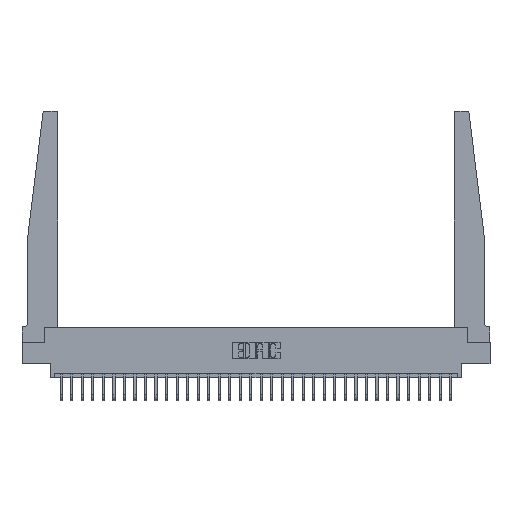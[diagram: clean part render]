
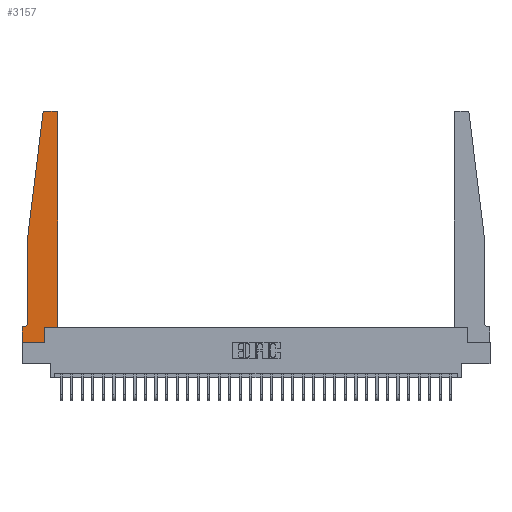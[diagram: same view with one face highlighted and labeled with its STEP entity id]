
A CAD part, top view. The second image highlights one B-rep face of the part: STEP entity #3157.
In plain terms, the highlighted planar face has unit normal (0, 0, 1).
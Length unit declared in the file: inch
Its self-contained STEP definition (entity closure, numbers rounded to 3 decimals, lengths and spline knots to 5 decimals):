
#404 = EDGE_CURVE ( 'NONE', #16977, #12662, #30665, .T. ) ;
#1570 = CIRCLE ( 'NONE', #20117, 0.05 ) ;
#1649 = CARTESIAN_POINT ( 'NONE',  ( 0.065, 0.2375, 0.37 ) ) ;
#1720 = CARTESIAN_POINT ( 'NONE',  ( 0.015, 0.2375, 0.37 ) ) ;
#2213 = CARTESIAN_POINT ( 'NONE',  ( 0., 0., 0.37 ) ) ;
#2411 = VECTOR ( 'NONE', #4899, 39.37008 ) ;
#2542 = ORIENTED_EDGE ( 'NONE', *, *, #15255, .T. ) ;
#2802 = EDGE_CURVE ( 'NONE', #7478, #3315, #29789, .T. ) ;
#3157 = ADVANCED_FACE ( 'NONE', ( #14568 ), #27684, .T. ) ;
#3315 = VERTEX_POINT ( 'NONE', #20793 ) ;
#3587 = DIRECTION ( 'NONE',  ( 0., 0., 1. ) ) ;
#3702 = VERTEX_POINT ( 'NONE', #26101 ) ;
#4328 = CARTESIAN_POINT ( 'NONE',  ( 0., 0.1875, 0.37 ) ) ;
#4753 = CARTESIAN_POINT ( 'NONE',  ( 0.065, 1.25, 0.37 ) ) ;
#4840 = VERTEX_POINT ( 'NONE', #12792 ) ;
#4899 = DIRECTION ( 'NONE',  ( -1., 0., 0. ) ) ;
#5077 = CARTESIAN_POINT ( 'NONE',  ( 0., 0.1875, 0.37 ) ) ;
#5295 = AXIS2_PLACEMENT_3D ( 'NONE', #22909, #23234, #8042 ) ;
#5657 = VERTEX_POINT ( 'NONE', #15448 ) ;
#6003 = LINE ( 'NONE', #20778, #17281 ) ;
#6250 = ORIENTED_EDGE ( 'NONE', *, *, #30817, .T. ) ;
#6309 = CARTESIAN_POINT ( 'NONE',  ( 0.27653, 2.72, 0.37 ) ) ;
#7261 = DIRECTION ( 'NONE',  ( 0., -1., 0. ) ) ;
#7462 = DIRECTION ( 'NONE',  ( 1., 0., 0. ) ) ;
#7478 = VERTEX_POINT ( 'NONE', #13219 ) ;
#8042 = DIRECTION ( 'NONE',  ( 1., 0., 0. ) ) ;
#9351 = EDGE_CURVE ( 'NONE', #14715, #16769, #27102, .T. ) ;
#9834 = VECTOR ( 'NONE', #16742, 39.37008 ) ;
#9995 = EDGE_CURVE ( 'NONE', #16769, #20593, #6003, .T. ) ;
#10140 = EDGE_CURVE ( 'NONE', #5657, #4840, #31924, .T. ) ;
#10900 = DIRECTION ( 'NONE',  ( 1., 0., 0. ) ) ;
#11083 = CARTESIAN_POINT ( 'NONE',  ( 0.425, 0.18, 0.37 ) ) ;
#11259 = ORIENTED_EDGE ( 'NONE', *, *, #29281, .T. ) ;
#11339 = ORIENTED_EDGE ( 'NONE', *, *, #404, .T. ) ;
#12044 = CIRCLE ( 'NONE', #19406, 0.03 ) ;
#12596 = VECTOR ( 'NONE', #30303, 39.37008 ) ;
#12662 = VERTEX_POINT ( 'NONE', #26445 ) ;
#12791 = DIRECTION ( 'NONE',  ( 0., 0., 1. ) ) ;
#12792 = CARTESIAN_POINT ( 'NONE',  ( 0.27653, 2.75, 0.37 ) ) ;
#12931 = CARTESIAN_POINT ( 'NONE',  ( 0.2605, 0.18, 0.37 ) ) ;
#12933 = DIRECTION ( 'NONE',  ( 0., -1., 0. ) ) ;
#13214 = EDGE_LOOP ( 'NONE', ( #26716, #2542, #11339, #28856, #30736, #14080, #29726, #18255, #19388, #6250, #16619, #11259 ) ) ;
#13219 = CARTESIAN_POINT ( 'NONE',  ( 0.425, 0.18, 0.37 ) ) ;
#13433 = VECTOR ( 'NONE', #19831, 39.37008 ) ;
#14080 = ORIENTED_EDGE ( 'NONE', *, *, #23127, .T. ) ;
#14568 = FACE_OUTER_BOUND ( 'NONE', #13214, .T. ) ;
#14636 = LINE ( 'NONE', #30090, #21653 ) ;
#14645 = CARTESIAN_POINT ( 'NONE',  ( 0.065, 0.1875, 0.37 ) ) ;
#14715 = VERTEX_POINT ( 'NONE', #4328 ) ;
#15255 = EDGE_CURVE ( 'NONE', #4840, #16977, #12044, .T. ) ;
#15448 = CARTESIAN_POINT ( 'NONE',  ( 0.395, 2.75, 0.37 ) ) ;
#15822 = AXIS2_PLACEMENT_3D ( 'NONE', #5077, #12791, #7462 ) ;
#15834 = DIRECTION ( 'NONE',  ( 1., 0., 0. ) ) ;
#15869 = VECTOR ( 'NONE', #15834, 39.37008 ) ;
#16035 = LINE ( 'NONE', #12931, #12596 ) ;
#16619 = ORIENTED_EDGE ( 'NONE', *, *, #2802, .T. ) ;
#16742 = DIRECTION ( 'NONE',  ( -1., 0., 0. ) ) ;
#16769 = VERTEX_POINT ( 'NONE', #18659 ) ;
#16977 = VERTEX_POINT ( 'NONE', #29431 ) ;
#17281 = VECTOR ( 'NONE', #23282, 39.37008 ) ;
#17885 = CIRCLE ( 'NONE', #5295, 0.03 ) ;
#18255 = ORIENTED_EDGE ( 'NONE', *, *, #9995, .T. ) ;
#18659 = CARTESIAN_POINT ( 'NONE',  ( 0., 0., 0.37 ) ) ;
#19321 = EDGE_CURVE ( 'NONE', #12662, #21809, #14636, .T. ) ;
#19388 = ORIENTED_EDGE ( 'NONE', *, *, #21782, .T. ) ;
#19406 = AXIS2_PLACEMENT_3D ( 'NONE', #6309, #3587, #10900 ) ;
#19831 = DIRECTION ( 'NONE',  ( 0., 1., 0. ) ) ;
#20117 = AXIS2_PLACEMENT_3D ( 'NONE', #1720, #31508, #28956 ) ;
#20463 = CARTESIAN_POINT ( 'NONE',  ( 0.2605, 0.18, 0.37 ) ) ;
#20593 = VERTEX_POINT ( 'NONE', #25349 ) ;
#20778 = CARTESIAN_POINT ( 'NONE',  ( 0., 0., 0.37 ) ) ;
#20793 = CARTESIAN_POINT ( 'NONE',  ( 0.425, 2.72, 0.37 ) ) ;
#21653 = VECTOR ( 'NONE', #12933, 39.37008 ) ;
#21782 = EDGE_CURVE ( 'NONE', #20593, #32049, #16035, .T. ) ;
#21809 = VERTEX_POINT ( 'NONE', #1649 ) ;
#22492 = LINE ( 'NONE', #11083, #15869 ) ;
#22909 = CARTESIAN_POINT ( 'NONE',  ( 0.395, 2.72, 0.37 ) ) ;
#23127 = EDGE_CURVE ( 'NONE', #3702, #14715, #23728, .T. ) ;
#23234 = DIRECTION ( 'NONE',  ( 0., 0., 1. ) ) ;
#23282 = DIRECTION ( 'NONE',  ( 1., 0., 0. ) ) ;
#23728 = LINE ( 'NONE', #14645, #2411 ) ;
#24320 = VECTOR ( 'NONE', #7261, 39.37008 ) ;
#24478 = VECTOR ( 'NONE', #28370, 39.37008 ) ;
#25349 = CARTESIAN_POINT ( 'NONE',  ( 0.2605, 0., 0.37 ) ) ;
#26101 = CARTESIAN_POINT ( 'NONE',  ( 0.015, 0.1875, 0.37 ) ) ;
#26445 = CARTESIAN_POINT ( 'NONE',  ( 0.065, 1.25, 0.37 ) ) ;
#26716 = ORIENTED_EDGE ( 'NONE', *, *, #10140, .T. ) ;
#27102 = LINE ( 'NONE', #2213, #24320 ) ;
#27684 = PLANE ( 'NONE',  #15822 ) ;
#28370 = DIRECTION ( 'NONE',  ( -0.122, -0.992, 0. ) ) ;
#28856 = ORIENTED_EDGE ( 'NONE', *, *, #19321, .T. ) ;
#28956 = DIRECTION ( 'NONE',  ( -1., 0., 0. ) ) ;
#29281 = EDGE_CURVE ( 'NONE', #3315, #5657, #17885, .T. ) ;
#29431 = CARTESIAN_POINT ( 'NONE',  ( 0.24675, 2.72367, 0.37 ) ) ;
#29599 = CARTESIAN_POINT ( 'NONE',  ( 0.425, 0.18, 0.37 ) ) ;
#29726 = ORIENTED_EDGE ( 'NONE', *, *, #9351, .T. ) ;
#29789 = LINE ( 'NONE', #29599, #13433 ) ;
#30078 = EDGE_CURVE ( 'NONE', #21809, #3702, #1570, .T. ) ;
#30090 = CARTESIAN_POINT ( 'NONE',  ( 0.065, 1.25, 0.37 ) ) ;
#30303 = DIRECTION ( 'NONE',  ( 0., 1., 0. ) ) ;
#30665 = LINE ( 'NONE', #4753, #24478 ) ;
#30736 = ORIENTED_EDGE ( 'NONE', *, *, #30078, .T. ) ;
#30817 = EDGE_CURVE ( 'NONE', #32049, #7478, #22492, .T. ) ;
#31508 = DIRECTION ( 'NONE',  ( 0., 0., -1. ) ) ;
#31591 = CARTESIAN_POINT ( 'NONE',  ( 0.25, 2.75, 0.37 ) ) ;
#31924 = LINE ( 'NONE', #31591, #9834 ) ;
#32049 = VERTEX_POINT ( 'NONE', #20463 ) ;
